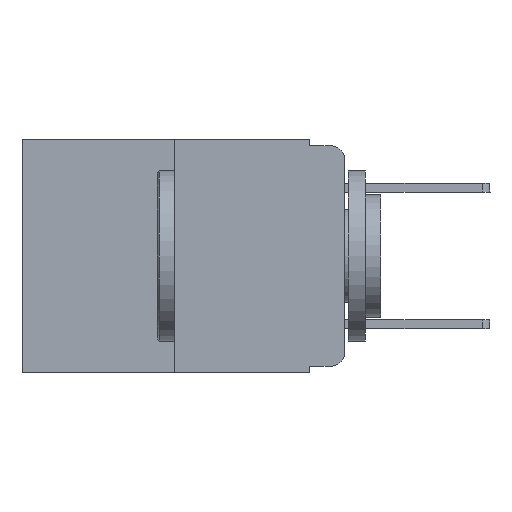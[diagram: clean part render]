
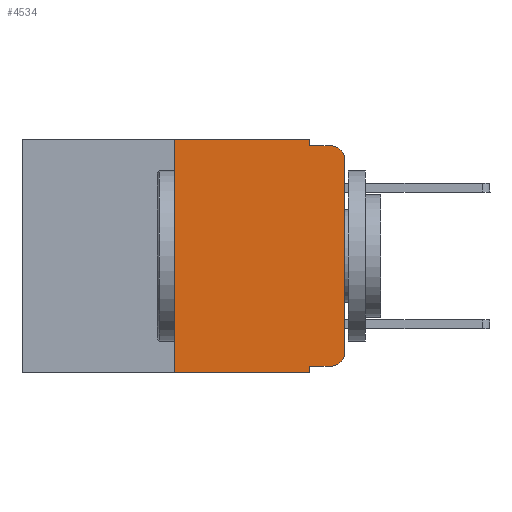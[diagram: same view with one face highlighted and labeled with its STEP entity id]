
A CAD part, left-side view. The second image highlights one B-rep face of the part: STEP entity #4534.
In plain terms, the highlighted planar face has unit normal (-1, 0, 0).
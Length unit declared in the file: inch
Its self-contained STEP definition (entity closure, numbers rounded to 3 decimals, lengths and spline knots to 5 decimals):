
#43 = CARTESIAN_POINT ( 'NONE',  ( 0., 0.473, 0. ) ) ;
#393 = CARTESIAN_POINT ( 'NONE',  ( 0., 0.473, 0. ) ) ;
#500 = LINE ( 'NONE', #10137, #12801 ) ;
#559 = EDGE_LOOP ( 'NONE', ( #1165, #7460, #4296, #12892, #7902, #7507, #10071, #13705, #13490, #7569 ) ) ;
#610 = CARTESIAN_POINT ( 'NONE',  ( 0., 0.051, -0.333 ) ) ;
#616 = DIRECTION ( 'NONE',  ( 0., 0., -1. ) ) ;
#798 = DIRECTION ( 'NONE',  ( -1., 0., 0. ) ) ;
#910 = CARTESIAN_POINT ( 'NONE',  ( 0., 0.051, 0. ) ) ;
#914 = LINE ( 'NONE', #3093, #11054 ) ;
#1165 = ORIENTED_EDGE ( 'NONE', *, *, #6838, .T. ) ;
#1722 = VERTEX_POINT ( 'NONE', #910 ) ;
#1784 = DIRECTION ( 'NONE',  ( 0., -1., 0. ) ) ;
#1793 = EDGE_CURVE ( 'NONE', #7824, #5025, #11277, .T. ) ;
#1865 = EDGE_CURVE ( 'NONE', #7824, #7574, #8631, .T. ) ;
#1895 = DIRECTION ( 'NONE',  ( 0., -1., 0. ) ) ;
#2081 = DIRECTION ( 'NONE',  ( 0., -1., 0. ) ) ;
#3093 = CARTESIAN_POINT ( 'NONE',  ( 0., 0.25, 0. ) ) ;
#3664 = EDGE_CURVE ( 'NONE', #5904, #7574, #500, .T. ) ;
#3671 = CIRCLE ( 'NONE', #11057, 0.02 ) ;
#4296 = ORIENTED_EDGE ( 'NONE', *, *, #5635, .F. ) ;
#4534 = ADVANCED_FACE ( 'NONE', ( #8148 ), #11215, .F. ) ;
#4616 = CARTESIAN_POINT ( 'NONE',  ( 0., 0., 0. ) ) ;
#4656 = CARTESIAN_POINT ( 'NONE',  ( 0., 0., -0.313 ) ) ;
#4704 = EDGE_CURVE ( 'NONE', #1722, #10697, #9819, .T. ) ;
#5025 = VERTEX_POINT ( 'NONE', #10216 ) ;
#5354 = VERTEX_POINT ( 'NONE', #9917 ) ;
#5473 = CARTESIAN_POINT ( 'NONE',  ( 0., 0.051, 0. ) ) ;
#5635 = EDGE_CURVE ( 'NONE', #10697, #5354, #11580, .T. ) ;
#5904 = VERTEX_POINT ( 'NONE', #10112 ) ;
#5930 = EDGE_CURVE ( 'NONE', #12152, #1722, #11353, .T. ) ;
#6046 = CARTESIAN_POINT ( 'NONE',  ( 0., 0.25, 0. ) ) ;
#6333 = CARTESIAN_POINT ( 'NONE',  ( 0., 0.051, -0.01 ) ) ;
#6580 = DIRECTION ( 'NONE',  ( 0., 0., -1. ) ) ;
#6592 = EDGE_CURVE ( 'NONE', #5025, #9196, #3671, .T. ) ;
#6838 = EDGE_CURVE ( 'NONE', #9196, #12895, #9948, .T. ) ;
#6911 = VECTOR ( 'NONE', #2081, 39.37008 ) ;
#6934 = DIRECTION ( 'NONE',  ( -1., 0., 0. ) ) ;
#6971 = DIRECTION ( 'NONE',  ( 0., 0., -1. ) ) ;
#7256 = VECTOR ( 'NONE', #8902, 39.37008 ) ;
#7279 = AXIS2_PLACEMENT_3D ( 'NONE', #9964, #6934, #8064 ) ;
#7460 = ORIENTED_EDGE ( 'NONE', *, *, #11389, .T. ) ;
#7507 = ORIENTED_EDGE ( 'NONE', *, *, #10737, .F. ) ;
#7569 = ORIENTED_EDGE ( 'NONE', *, *, #6592, .T. ) ;
#7574 = VERTEX_POINT ( 'NONE', #13753 ) ;
#7579 = DIRECTION ( 'NONE',  ( 0., 0., -1. ) ) ;
#7636 = CARTESIAN_POINT ( 'NONE',  ( 0., 0., -0.03 ) ) ;
#7679 = AXIS2_PLACEMENT_3D ( 'NONE', #393, #13528, #616 ) ;
#7805 = CARTESIAN_POINT ( 'NONE',  ( 0., 0.051, -0.333 ) ) ;
#7824 = VERTEX_POINT ( 'NONE', #7805 ) ;
#7902 = ORIENTED_EDGE ( 'NONE', *, *, #5930, .F. ) ;
#7911 = VECTOR ( 'NONE', #12839, 39.37008 ) ;
#8064 = DIRECTION ( 'NONE',  ( 0., 0., -1. ) ) ;
#8145 = VECTOR ( 'NONE', #6580, 39.37008 ) ;
#8148 = FACE_OUTER_BOUND ( 'NONE', #559, .T. ) ;
#8379 = CARTESIAN_POINT ( 'NONE',  ( 0., 0.051, -0.01 ) ) ;
#8631 = LINE ( 'NONE', #5473, #10946 ) ;
#8902 = DIRECTION ( 'NONE',  ( 0., 0., 1. ) ) ;
#9196 = VERTEX_POINT ( 'NONE', #4656 ) ;
#9359 = DIRECTION ( 'NONE',  ( 0., 0., 1. ) ) ;
#9819 = LINE ( 'NONE', #11762, #8145 ) ;
#9917 = CARTESIAN_POINT ( 'NONE',  ( 0., 0.02, -0.01 ) ) ;
#9948 = LINE ( 'NONE', #4616, #7256 ) ;
#9964 = CARTESIAN_POINT ( 'NONE',  ( 0., 0.02, -0.03 ) ) ;
#10071 = ORIENTED_EDGE ( 'NONE', *, *, #3664, .T. ) ;
#10112 = CARTESIAN_POINT ( 'NONE',  ( 0., 0.25, -0.343 ) ) ;
#10137 = CARTESIAN_POINT ( 'NONE',  ( 0., 0.473, -0.343 ) ) ;
#10216 = CARTESIAN_POINT ( 'NONE',  ( 0., 0.02, -0.333 ) ) ;
#10337 = CARTESIAN_POINT ( 'NONE',  ( 0., 0.02, -0.313 ) ) ;
#10697 = VERTEX_POINT ( 'NONE', #8379 ) ;
#10737 = EDGE_CURVE ( 'NONE', #5904, #12152, #914, .T. ) ;
#10869 = CIRCLE ( 'NONE', #7279, 0.02 ) ;
#10946 = VECTOR ( 'NONE', #7579, 39.37008 ) ;
#11054 = VECTOR ( 'NONE', #9359, 39.37008 ) ;
#11057 = AXIS2_PLACEMENT_3D ( 'NONE', #10337, #798, #6971 ) ;
#11215 = PLANE ( 'NONE',  #7679 ) ;
#11277 = LINE ( 'NONE', #610, #6911 ) ;
#11353 = LINE ( 'NONE', #43, #12584 ) ;
#11389 = EDGE_CURVE ( 'NONE', #12895, #5354, #10869, .T. ) ;
#11580 = LINE ( 'NONE', #6333, #7911 ) ;
#11762 = CARTESIAN_POINT ( 'NONE',  ( 0., 0.051, 0. ) ) ;
#12152 = VERTEX_POINT ( 'NONE', #6046 ) ;
#12584 = VECTOR ( 'NONE', #1895, 39.37008 ) ;
#12801 = VECTOR ( 'NONE', #1784, 39.37008 ) ;
#12839 = DIRECTION ( 'NONE',  ( 0., -1., 0. ) ) ;
#12892 = ORIENTED_EDGE ( 'NONE', *, *, #4704, .F. ) ;
#12895 = VERTEX_POINT ( 'NONE', #7636 ) ;
#13490 = ORIENTED_EDGE ( 'NONE', *, *, #1793, .T. ) ;
#13528 = DIRECTION ( 'NONE',  ( 1., 0., 0. ) ) ;
#13705 = ORIENTED_EDGE ( 'NONE', *, *, #1865, .F. ) ;
#13753 = CARTESIAN_POINT ( 'NONE',  ( 0., 0.051, -0.343 ) ) ;
